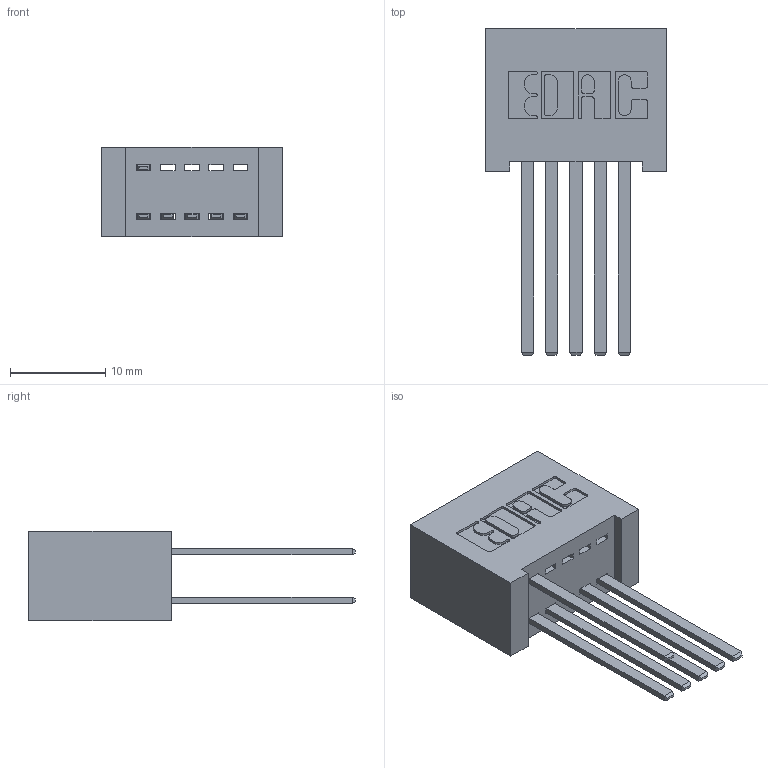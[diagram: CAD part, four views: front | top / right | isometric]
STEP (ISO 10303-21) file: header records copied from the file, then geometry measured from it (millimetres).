
FILE_DESCRIPTION (( 'STEP AP203' ), '1' );
FILE_NAME ('342-010-544-201.STEP', '2018-08-10T13:49:59', ( '' ), ( '' ), 'SwSTEP 2.0', 'SolidWorks 2016', '' );
FILE_SCHEMA (( 'CONFIG_CONTROL_DESIGN' ));
Length unit declared in the file: inch
Products named in the file (3): 342-010-544-201; 342 Part_Lugless; 345-292-001_345-293-144
Assembly tree (7 placements, depth 2):
  342-010-544-201
    342 Part_Lugless
    345-292-001_345-293-144  x6
Bounding box: 18.95 x 34.3 x 9.4 mm (x, y, z)
Volume: 2015 mm3; surface area: 2848.4 mm2
Topology: 7 solids, 7 shells, 402 faces, 1181 edges, 778 vertices
Faces by surface type: plane 278, cylinder 124
Entity records: 7281 total; most frequent: CARTESIAN_POINT 1262, ORIENTED_EDGE 1202, DIRECTION 1129, EDGE_CURVE 601, LINE 485, VECTOR 485, VERTEX_POINT 398, AXIS2_PLACEMENT_3D 322
